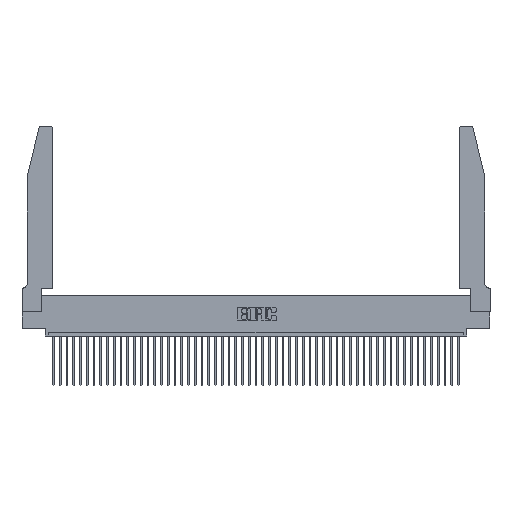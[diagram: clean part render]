
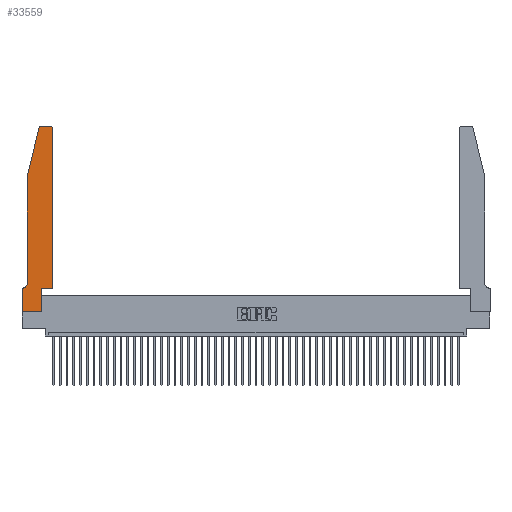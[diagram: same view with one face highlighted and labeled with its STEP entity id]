
A CAD part, top view. The second image highlights one B-rep face of the part: STEP entity #33559.
In plain terms, the highlighted planar face has unit normal (0, 0, 1).
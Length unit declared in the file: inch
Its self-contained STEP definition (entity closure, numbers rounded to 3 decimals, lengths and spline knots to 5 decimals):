
#4 = VERTEX_POINT ( 'NONE', #42135 ) ;
#405 = AXIS2_PLACEMENT_3D ( 'NONE', #22662, #22214, #26131 ) ;
#2001 = FACE_OUTER_BOUND ( 'NONE', #38853, .T. ) ;
#2051 = VECTOR ( 'NONE', #35683, 39.37008 ) ;
#2241 = VECTOR ( 'NONE', #6665, 39.37008 ) ;
#2261 = DIRECTION ( 'NONE',  ( 0., 0., 1. ) ) ;
#2648 = CARTESIAN_POINT ( 'NONE',  ( 0., 0., 0.37 ) ) ;
#3017 = EDGE_CURVE ( 'NONE', #41296, #22534, #9353, .T. ) ;
#3146 = VERTEX_POINT ( 'NONE', #17607 ) ;
#3482 = VERTEX_POINT ( 'NONE', #13256 ) ;
#3881 = LINE ( 'NONE', #14298, #7397 ) ;
#4331 = VERTEX_POINT ( 'NONE', #12897 ) ;
#4438 = DIRECTION ( 'NONE',  ( 1., 0., 0. ) ) ;
#4936 = CIRCLE ( 'NONE', #21653, 0.03 ) ;
#4999 = VECTOR ( 'NONE', #32950, 39.37008 ) ;
#5148 = VERTEX_POINT ( 'NONE', #21907 ) ;
#6665 = DIRECTION ( 'NONE',  ( -0.239, -0.971, 0. ) ) ;
#7355 = EDGE_CURVE ( 'NONE', #4, #3146, #46328, .T. ) ;
#7397 = VECTOR ( 'NONE', #28855, 39.37008 ) ;
#7493 = AXIS2_PLACEMENT_3D ( 'NONE', #18717, #20015, #41789 ) ;
#8724 = AXIS2_PLACEMENT_3D ( 'NONE', #35634, #2261, #9731 ) ;
#9353 = LINE ( 'NONE', #35007, #22209 ) ;
#9731 = DIRECTION ( 'NONE',  ( 1., 0., 0. ) ) ;
#9755 = VECTOR ( 'NONE', #11956, 39.37008 ) ;
#10263 = VECTOR ( 'NONE', #16733, 39.37008 ) ;
#10457 = ORIENTED_EDGE ( 'NONE', *, *, #40853, .T. ) ;
#10619 = ORIENTED_EDGE ( 'NONE', *, *, #25436, .T. ) ;
#10918 = VERTEX_POINT ( 'NONE', #32849 ) ;
#11218 = EDGE_CURVE ( 'NONE', #3482, #4331, #27276, .T. ) ;
#11956 = DIRECTION ( 'NONE',  ( 0., 1., 0. ) ) ;
#12375 = DIRECTION ( 'NONE',  ( 0., 0., 1. ) ) ;
#12449 = EDGE_CURVE ( 'NONE', #3146, #3482, #40747, .T. ) ;
#12897 = CARTESIAN_POINT ( 'NONE',  ( 0.0755, 2., 0.37 ) ) ;
#13256 = CARTESIAN_POINT ( 'NONE',  ( 0.25487, 2.72718, 0.37 ) ) ;
#13574 = EDGE_CURVE ( 'NONE', #5148, #10918, #3881, .T. ) ;
#13659 = ORIENTED_EDGE ( 'NONE', *, *, #12449, .T. ) ;
#13954 = DIRECTION ( 'NONE',  ( 0., 1., 0. ) ) ;
#14298 = CARTESIAN_POINT ( 'NONE',  ( 0.4505, 0.35, 0.37 ) ) ;
#14532 = DIRECTION ( 'NONE',  ( 0., -1., 0. ) ) ;
#15021 = VERTEX_POINT ( 'NONE', #34052 ) ;
#16106 = CARTESIAN_POINT ( 'NONE',  ( 0.4505, 2.72, 0.37 ) ) ;
#16594 = LINE ( 'NONE', #39740, #2051 ) ;
#16733 = DIRECTION ( 'NONE',  ( -1., 0., 0. ) ) ;
#17607 = CARTESIAN_POINT ( 'NONE',  ( 0.284, 2.75, 0.37 ) ) ;
#18028 = EDGE_CURVE ( 'NONE', #22534, #5148, #33158, .T. ) ;
#18271 = VERTEX_POINT ( 'NONE', #16106 ) ;
#18717 = CARTESIAN_POINT ( 'NONE',  ( 0., 0.35, 0.37 ) ) ;
#19422 = ORIENTED_EDGE ( 'NONE', *, *, #29348, .T. ) ;
#20015 = DIRECTION ( 'NONE',  ( 0., 0., 1. ) ) ;
#21134 = ORIENTED_EDGE ( 'NONE', *, *, #11218, .T. ) ;
#21344 = CARTESIAN_POINT ( 'NONE',  ( 0.2865, 0., 0.37 ) ) ;
#21653 = AXIS2_PLACEMENT_3D ( 'NONE', #22859, #12375, #4438 ) ;
#21907 = CARTESIAN_POINT ( 'NONE',  ( 0.2865, 0.35, 0.37 ) ) ;
#22053 = CARTESIAN_POINT ( 'NONE',  ( 0., 0., 0.37 ) ) ;
#22209 = VECTOR ( 'NONE', #38079, 39.37008 ) ;
#22214 = DIRECTION ( 'NONE',  ( 0., 0., -1. ) ) ;
#22534 = VERTEX_POINT ( 'NONE', #21344 ) ;
#22662 = CARTESIAN_POINT ( 'NONE',  ( 0.0055, 0.42, 0.37 ) ) ;
#22831 = ORIENTED_EDGE ( 'NONE', *, *, #47247, .T. ) ;
#22859 = CARTESIAN_POINT ( 'NONE',  ( 0.4205, 2.72, 0.37 ) ) ;
#25094 = CARTESIAN_POINT ( 'NONE',  ( 0.2865, 0.35, 0.37 ) ) ;
#25383 = CARTESIAN_POINT ( 'NONE',  ( 0.0755, 2., 0.37 ) ) ;
#25436 = EDGE_CURVE ( 'NONE', #18271, #4, #4936, .T. ) ;
#26131 = DIRECTION ( 'NONE',  ( -1., 0., 0. ) ) ;
#27276 = LINE ( 'NONE', #43594, #2241 ) ;
#28089 = VERTEX_POINT ( 'NONE', #38557 ) ;
#28855 = DIRECTION ( 'NONE',  ( 1., 0., 0. ) ) ;
#29155 = CIRCLE ( 'NONE', #405, 0.07 ) ;
#29348 = EDGE_CURVE ( 'NONE', #28089, #15021, #29155, .T. ) ;
#29653 = VECTOR ( 'NONE', #13954, 39.37008 ) ;
#30787 = ORIENTED_EDGE ( 'NONE', *, *, #31344, .T. ) ;
#30791 = ORIENTED_EDGE ( 'NONE', *, *, #7355, .T. ) ;
#30792 = VECTOR ( 'NONE', #14532, 39.37008 ) ;
#31344 = EDGE_CURVE ( 'NONE', #10918, #18271, #34190, .T. ) ;
#32529 = EDGE_CURVE ( 'NONE', #15021, #43176, #16594, .T. ) ;
#32849 = CARTESIAN_POINT ( 'NONE',  ( 0.4505, 0.35, 0.37 ) ) ;
#32950 = DIRECTION ( 'NONE',  ( 0., -1., 0. ) ) ;
#33158 = LINE ( 'NONE', #25094, #29653 ) ;
#33381 = LINE ( 'NONE', #25383, #30792 ) ;
#33426 = ORIENTED_EDGE ( 'NONE', *, *, #13574, .T. ) ;
#33559 = ADVANCED_FACE ( 'NONE', ( #2001 ), #34311, .T. ) ;
#34052 = CARTESIAN_POINT ( 'NONE',  ( 0.0055, 0.35, 0.37 ) ) ;
#34190 = LINE ( 'NONE', #34300, #9755 ) ;
#34300 = CARTESIAN_POINT ( 'NONE',  ( 0.4505, 0.35, 0.37 ) ) ;
#34311 = PLANE ( 'NONE',  #7493 ) ;
#34653 = ORIENTED_EDGE ( 'NONE', *, *, #3017, .T. ) ;
#35007 = CARTESIAN_POINT ( 'NONE',  ( 0., 0., 0.37 ) ) ;
#35634 = CARTESIAN_POINT ( 'NONE',  ( 0.284, 2.72, 0.37 ) ) ;
#35683 = DIRECTION ( 'NONE',  ( -1., 0., 0. ) ) ;
#38079 = DIRECTION ( 'NONE',  ( 1., 0., 0. ) ) ;
#38170 = LINE ( 'NONE', #22053, #4999 ) ;
#38557 = CARTESIAN_POINT ( 'NONE',  ( 0.0755, 0.42, 0.37 ) ) ;
#38853 = EDGE_LOOP ( 'NONE', ( #30791, #13659, #21134, #22831, #19422, #48078, #10457, #34653, #45649, #33426, #30787, #10619 ) ) ;
#39740 = CARTESIAN_POINT ( 'NONE',  ( 0.0755, 0.35, 0.37 ) ) ;
#40235 = CARTESIAN_POINT ( 'NONE',  ( 0., 0.35, 0.37 ) ) ;
#40747 = CIRCLE ( 'NONE', #8724, 0.03 ) ;
#40853 = EDGE_CURVE ( 'NONE', #43176, #41296, #38170, .T. ) ;
#41296 = VERTEX_POINT ( 'NONE', #2648 ) ;
#41789 = DIRECTION ( 'NONE',  ( 1., 0., 0. ) ) ;
#42135 = CARTESIAN_POINT ( 'NONE',  ( 0.4205, 2.75, 0.37 ) ) ;
#42472 = CARTESIAN_POINT ( 'NONE',  ( 0.2605, 2.75, 0.37 ) ) ;
#43176 = VERTEX_POINT ( 'NONE', #40235 ) ;
#43594 = CARTESIAN_POINT ( 'NONE',  ( 0.0755, 2., 0.37 ) ) ;
#45649 = ORIENTED_EDGE ( 'NONE', *, *, #18028, .T. ) ;
#46328 = LINE ( 'NONE', #42472, #10263 ) ;
#47247 = EDGE_CURVE ( 'NONE', #4331, #28089, #33381, .T. ) ;
#48078 = ORIENTED_EDGE ( 'NONE', *, *, #32529, .T. ) ;
